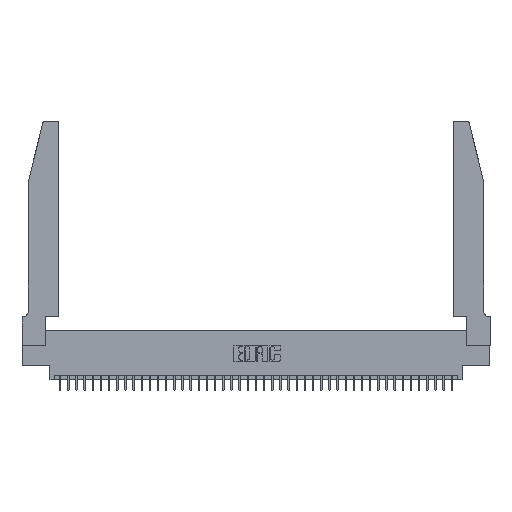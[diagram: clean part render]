
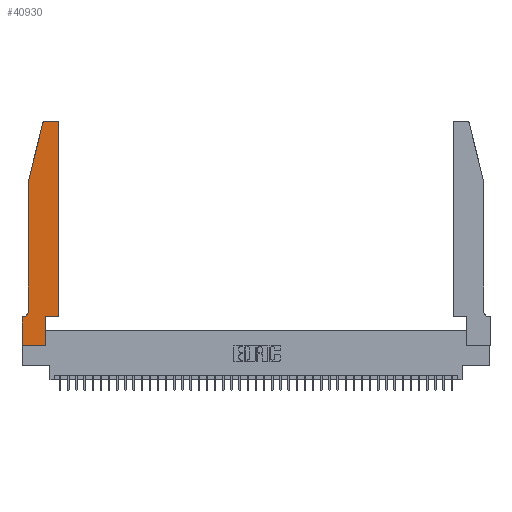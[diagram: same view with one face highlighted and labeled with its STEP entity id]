
A CAD part, top view. The second image highlights one B-rep face of the part: STEP entity #40930.
In plain terms, the highlighted planar face has unit normal (0, 0, 1).
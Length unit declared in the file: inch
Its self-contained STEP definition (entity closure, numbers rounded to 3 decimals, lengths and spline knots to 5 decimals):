
#1330 = CARTESIAN_POINT ( 'NONE',  ( 0.25487, 2.72718, 0.37 ) ) ;
#1710 = LINE ( 'NONE', #8779, #25818 ) ;
#1883 = CARTESIAN_POINT ( 'NONE',  ( 0.284, 2.75, 0.37 ) ) ;
#1952 = ORIENTED_EDGE ( 'NONE', *, *, #23649, .T. ) ;
#1986 = LINE ( 'NONE', #12274, #10442 ) ;
#2307 = DIRECTION ( 'NONE',  ( -1., 0., 0. ) ) ;
#2919 = DIRECTION ( 'NONE',  ( 1., 0., 0. ) ) ;
#3929 = FACE_OUTER_BOUND ( 'NONE', #5931, .T. ) ;
#3942 = EDGE_CURVE ( 'NONE', #34446, #24390, #26523, .T. ) ;
#4805 = DIRECTION ( 'NONE',  ( 1., 0., 0. ) ) ;
#5931 = EDGE_LOOP ( 'NONE', ( #10935, #25613, #32079, #23199, #1952, #34136, #19084, #16703, #27093, #13215, #15383, #20757 ) ) ;
#7686 = VERTEX_POINT ( 'NONE', #12178 ) ;
#8281 = EDGE_CURVE ( 'NONE', #23833, #36664, #8374, .T. ) ;
#8374 = LINE ( 'NONE', #37652, #40339 ) ;
#8779 = CARTESIAN_POINT ( 'NONE',  ( 0.2605, 2.75, 0.37 ) ) ;
#9803 = CARTESIAN_POINT ( 'NONE',  ( 0.0755, 2., 0.37 ) ) ;
#10442 = VECTOR ( 'NONE', #41342, 39.37008 ) ;
#10651 = CARTESIAN_POINT ( 'NONE',  ( 0.0055, 0.35, 0.37 ) ) ;
#10817 = DIRECTION ( 'NONE',  ( 1., 0., 0. ) ) ;
#10935 = ORIENTED_EDGE ( 'NONE', *, *, #36215, .T. ) ;
#11251 = VERTEX_POINT ( 'NONE', #11958 ) ;
#11281 = EDGE_CURVE ( 'NONE', #41747, #11251, #15830, .T. ) ;
#11515 = EDGE_CURVE ( 'NONE', #33551, #15693, #37735, .T. ) ;
#11958 = CARTESIAN_POINT ( 'NONE',  ( 0.0755, 2., 0.37 ) ) ;
#12178 = CARTESIAN_POINT ( 'NONE',  ( 0.4205, 2.75, 0.37 ) ) ;
#12274 = CARTESIAN_POINT ( 'NONE',  ( 0.0755, 2., 0.37 ) ) ;
#12376 = VECTOR ( 'NONE', #21576, 39.37008 ) ;
#12593 = DIRECTION ( 'NONE',  ( -0.239, -0.971, 0. ) ) ;
#13096 = AXIS2_PLACEMENT_3D ( 'NONE', #37312, #37108, #4805 ) ;
#13215 = ORIENTED_EDGE ( 'NONE', *, *, #28411, .T. ) ;
#13262 = VERTEX_POINT ( 'NONE', #18791 ) ;
#13686 = CARTESIAN_POINT ( 'NONE',  ( 0.2865, 0., 0.37 ) ) ;
#14062 = VECTOR ( 'NONE', #23251, 39.37008 ) ;
#14659 = VECTOR ( 'NONE', #14924, 39.37008 ) ;
#14810 = DIRECTION ( 'NONE',  ( -1., 0., 0. ) ) ;
#14924 = DIRECTION ( 'NONE',  ( -1., 0., 0. ) ) ;
#15383 = ORIENTED_EDGE ( 'NONE', *, *, #3942, .T. ) ;
#15693 = VERTEX_POINT ( 'NONE', #23151 ) ;
#15820 = CARTESIAN_POINT ( 'NONE',  ( 0., 0., 0.37 ) ) ;
#15830 = LINE ( 'NONE', #9803, #18825 ) ;
#16703 = ORIENTED_EDGE ( 'NONE', *, *, #35443, .T. ) ;
#16706 = CIRCLE ( 'NONE', #40732, 0.03 ) ;
#16856 = PLANE ( 'NONE',  #19041 ) ;
#17237 = CARTESIAN_POINT ( 'NONE',  ( 0., 0.35, 0.37 ) ) ;
#18140 = CIRCLE ( 'NONE', #18821, 0.07 ) ;
#18144 = LINE ( 'NONE', #37930, #12376 ) ;
#18791 = CARTESIAN_POINT ( 'NONE',  ( 0.0755, 0.42, 0.37 ) ) ;
#18821 = AXIS2_PLACEMENT_3D ( 'NONE', #22303, #38639, #2307 ) ;
#18825 = VECTOR ( 'NONE', #12593, 39.37008 ) ;
#19041 = AXIS2_PLACEMENT_3D ( 'NONE', #17237, #26313, #10817 ) ;
#19084 = ORIENTED_EDGE ( 'NONE', *, *, #37411, .T. ) ;
#19089 = LINE ( 'NONE', #22317, #23111 ) ;
#20670 = CIRCLE ( 'NONE', #13096, 0.03 ) ;
#20757 = ORIENTED_EDGE ( 'NONE', *, *, #33696, .T. ) ;
#21576 = DIRECTION ( 'NONE',  ( 1., 0., 0. ) ) ;
#22303 = CARTESIAN_POINT ( 'NONE',  ( 0.0055, 0.42, 0.37 ) ) ;
#22317 = CARTESIAN_POINT ( 'NONE',  ( 0., 0., 0.37 ) ) ;
#23111 = VECTOR ( 'NONE', #32258, 39.37008 ) ;
#23151 = CARTESIAN_POINT ( 'NONE',  ( 0., 0.35, 0.37 ) ) ;
#23199 = ORIENTED_EDGE ( 'NONE', *, *, #30003, .T. ) ;
#23251 = DIRECTION ( 'NONE',  ( 0., 1., 0. ) ) ;
#23649 = EDGE_CURVE ( 'NONE', #13262, #33551, #18140, .T. ) ;
#23833 = VERTEX_POINT ( 'NONE', #13686 ) ;
#24390 = VERTEX_POINT ( 'NONE', #33535 ) ;
#25613 = ORIENTED_EDGE ( 'NONE', *, *, #29381, .T. ) ;
#25818 = VECTOR ( 'NONE', #14810, 39.37008 ) ;
#26313 = DIRECTION ( 'NONE',  ( 0., 0., 1. ) ) ;
#26514 = VERTEX_POINT ( 'NONE', #39217 ) ;
#26523 = LINE ( 'NONE', #33406, #14062 ) ;
#27093 = ORIENTED_EDGE ( 'NONE', *, *, #8281, .T. ) ;
#27514 = CARTESIAN_POINT ( 'NONE',  ( 0.4505, 0.35, 0.37 ) ) ;
#27841 = DIRECTION ( 'NONE',  ( 1., 0., 0. ) ) ;
#28067 = CARTESIAN_POINT ( 'NONE',  ( 0.2865, 0.35, 0.37 ) ) ;
#28411 = EDGE_CURVE ( 'NONE', #36664, #34446, #18144, .T. ) ;
#29381 = EDGE_CURVE ( 'NONE', #39281, #41747, #20670, .T. ) ;
#30003 = EDGE_CURVE ( 'NONE', #11251, #13262, #1986, .T. ) ;
#31045 = DIRECTION ( 'NONE',  ( 0., 0., 1. ) ) ;
#31278 = CARTESIAN_POINT ( 'NONE',  ( 0.4205, 2.72, 0.37 ) ) ;
#32079 = ORIENTED_EDGE ( 'NONE', *, *, #11281, .T. ) ;
#32258 = DIRECTION ( 'NONE',  ( 0., -1., 0. ) ) ;
#32638 = LINE ( 'NONE', #15820, #39530 ) ;
#33406 = CARTESIAN_POINT ( 'NONE',  ( 0.4505, 0.35, 0.37 ) ) ;
#33535 = CARTESIAN_POINT ( 'NONE',  ( 0.4505, 2.72, 0.37 ) ) ;
#33551 = VERTEX_POINT ( 'NONE', #10651 ) ;
#33696 = EDGE_CURVE ( 'NONE', #24390, #7686, #16706, .T. ) ;
#34136 = ORIENTED_EDGE ( 'NONE', *, *, #11515, .T. ) ;
#34446 = VERTEX_POINT ( 'NONE', #27514 ) ;
#35443 = EDGE_CURVE ( 'NONE', #26514, #23833, #32638, .T. ) ;
#36215 = EDGE_CURVE ( 'NONE', #7686, #39281, #1710, .T. ) ;
#36664 = VERTEX_POINT ( 'NONE', #28067 ) ;
#37108 = DIRECTION ( 'NONE',  ( 0., 0., 1. ) ) ;
#37312 = CARTESIAN_POINT ( 'NONE',  ( 0.284, 2.72, 0.37 ) ) ;
#37411 = EDGE_CURVE ( 'NONE', #15693, #26514, #19089, .T. ) ;
#37529 = CARTESIAN_POINT ( 'NONE',  ( 0.0755, 0.35, 0.37 ) ) ;
#37652 = CARTESIAN_POINT ( 'NONE',  ( 0.2865, 0.35, 0.37 ) ) ;
#37735 = LINE ( 'NONE', #37529, #14659 ) ;
#37930 = CARTESIAN_POINT ( 'NONE',  ( 0.4505, 0.35, 0.37 ) ) ;
#38639 = DIRECTION ( 'NONE',  ( 0., 0., -1. ) ) ;
#39217 = CARTESIAN_POINT ( 'NONE',  ( 0., 0., 0.37 ) ) ;
#39281 = VERTEX_POINT ( 'NONE', #1883 ) ;
#39530 = VECTOR ( 'NONE', #2919, 39.37008 ) ;
#40339 = VECTOR ( 'NONE', #41094, 39.37008 ) ;
#40732 = AXIS2_PLACEMENT_3D ( 'NONE', #31278, #31045, #27841 ) ;
#40930 = ADVANCED_FACE ( 'NONE', ( #3929 ), #16856, .T. ) ;
#41094 = DIRECTION ( 'NONE',  ( 0., 1., 0. ) ) ;
#41342 = DIRECTION ( 'NONE',  ( 0., -1., 0. ) ) ;
#41747 = VERTEX_POINT ( 'NONE', #1330 ) ;
